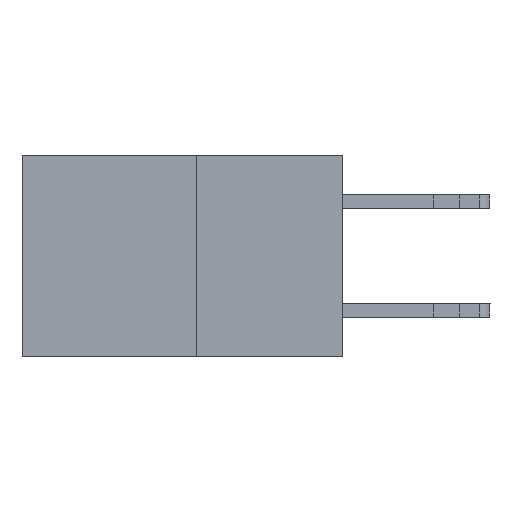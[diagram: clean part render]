
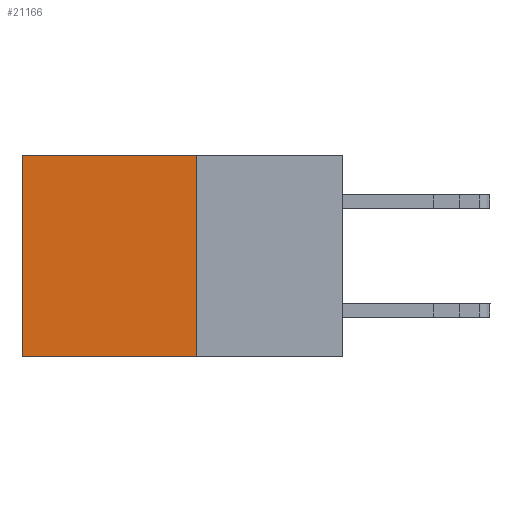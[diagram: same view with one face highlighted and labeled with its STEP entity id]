
A CAD part, left-side view. The second image highlights one B-rep face of the part: STEP entity #21166.
In plain terms, the highlighted planar face has unit normal (-1, 0, 0).
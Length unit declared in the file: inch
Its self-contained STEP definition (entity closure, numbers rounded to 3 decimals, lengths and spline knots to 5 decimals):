
#251 = CARTESIAN_POINT ( 'NONE',  ( 0.277, 0.27, -0.37 ) ) ;
#1019 = CARTESIAN_POINT ( 'NONE',  ( 0.277, 0.27, -0.37 ) ) ;
#2532 = CARTESIAN_POINT ( 'NONE',  ( 0.277, 0.27, -0.37 ) ) ;
#2621 = DIRECTION ( 'NONE',  ( 1., 0., 0. ) ) ;
#3121 = CARTESIAN_POINT ( 'NONE',  ( 0.277, 0.27, -0.37 ) ) ;
#3564 = VERTEX_POINT ( 'NONE', #20111 ) ;
#3943 = CARTESIAN_POINT ( 'NONE',  ( 0.277, 0.59, -0.37 ) ) ;
#4379 = VERTEX_POINT ( 'NONE', #24921 ) ;
#6152 = VECTOR ( 'NONE', #26568, 39.37008 ) ;
#8732 = DIRECTION ( 'NONE',  ( 0., 0., -1. ) ) ;
#9621 = EDGE_CURVE ( 'NONE', #21828, #11396, #23062, .T. ) ;
#10221 = LINE ( 'NONE', #3121, #20115 ) ;
#10948 = DIRECTION ( 'NONE',  ( 0., 1., 0. ) ) ;
#11259 = EDGE_CURVE ( 'NONE', #3564, #4379, #17376, .T. ) ;
#11321 = CARTESIAN_POINT ( 'NONE',  ( 0.277, 0.59, -0.37 ) ) ;
#11396 = VERTEX_POINT ( 'NONE', #11321 ) ;
#11533 = EDGE_LOOP ( 'NONE', ( #15475, #23757, #20773, #12034 ) ) ;
#11813 = VECTOR ( 'NONE', #10948, 39.37008 ) ;
#12034 = ORIENTED_EDGE ( 'NONE', *, *, #11259, .T. ) ;
#15470 = PLANE ( 'NONE',  #26557 ) ;
#15475 = ORIENTED_EDGE ( 'NONE', *, *, #23368, .T. ) ;
#16492 = VECTOR ( 'NONE', #8732, 39.37008 ) ;
#17175 = EDGE_CURVE ( 'NONE', #3564, #21828, #10221, .T. ) ;
#17376 = LINE ( 'NONE', #23538, #11813 ) ;
#17592 = DIRECTION ( 'NONE',  ( 0., 0., -1. ) ) ;
#20111 = CARTESIAN_POINT ( 'NONE',  ( 0.277, 0.27, 0. ) ) ;
#20115 = VECTOR ( 'NONE', #20206, 39.37008 ) ;
#20206 = DIRECTION ( 'NONE',  ( 0., 0., -1. ) ) ;
#20773 = ORIENTED_EDGE ( 'NONE', *, *, #17175, .F. ) ;
#21166 = ADVANCED_FACE ( 'NONE', ( #27138 ), #15470, .F. ) ;
#21828 = VERTEX_POINT ( 'NONE', #251 ) ;
#22321 = LINE ( 'NONE', #3943, #16492 ) ;
#23062 = LINE ( 'NONE', #1019, #6152 ) ;
#23368 = EDGE_CURVE ( 'NONE', #4379, #11396, #22321, .T. ) ;
#23538 = CARTESIAN_POINT ( 'NONE',  ( 0.277, 0.27, 0. ) ) ;
#23757 = ORIENTED_EDGE ( 'NONE', *, *, #9621, .F. ) ;
#24921 = CARTESIAN_POINT ( 'NONE',  ( 0.277, 0.59, 0. ) ) ;
#26557 = AXIS2_PLACEMENT_3D ( 'NONE', #2532, #2621, #17592 ) ;
#26568 = DIRECTION ( 'NONE',  ( 0., 1., 0. ) ) ;
#27138 = FACE_OUTER_BOUND ( 'NONE', #11533, .T. ) ;
